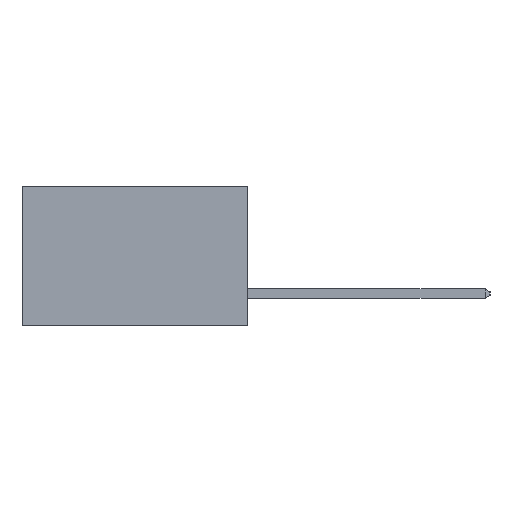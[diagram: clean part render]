
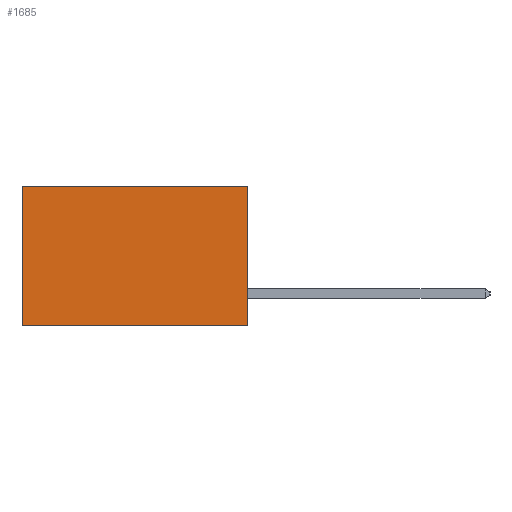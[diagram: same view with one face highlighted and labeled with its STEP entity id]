
A CAD part, left-side view. The second image highlights one B-rep face of the part: STEP entity #1685.
In plain terms, the highlighted planar face has unit normal (-1, 0, 0).
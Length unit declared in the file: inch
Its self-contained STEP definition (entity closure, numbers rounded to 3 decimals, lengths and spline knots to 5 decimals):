
#206 = VERTEX_POINT ( 'NONE', #11413 ) ;
#1685 = ADVANCED_FACE ( 'NONE', ( #15598 ), #6533, .F. ) ;
#3555 = VERTEX_POINT ( 'NONE', #18419 ) ;
#3852 = EDGE_CURVE ( 'NONE', #3555, #15900, #16230, .T. ) ;
#4130 = EDGE_CURVE ( 'NONE', #206, #18796, #12175, .T. ) ;
#6242 = DIRECTION ( 'NONE',  ( 1., 0., 0. ) ) ;
#6412 = DIRECTION ( 'NONE',  ( 0., 0., -1. ) ) ;
#6506 = CARTESIAN_POINT ( 'NONE',  ( 0.2615, 0., -0.37 ) ) ;
#6533 = PLANE ( 'NONE',  #6864 ) ;
#6864 = AXIS2_PLACEMENT_3D ( 'NONE', #6506, #6242, #6412 ) ;
#7263 = CARTESIAN_POINT ( 'NONE',  ( 0.2615, 0., -0.37 ) ) ;
#7342 = DIRECTION ( 'NONE',  ( 0., 0., -1. ) ) ;
#8049 = VECTOR ( 'NONE', #7342, 39.37008 ) ;
#8057 = VECTOR ( 'NONE', #14753, 39.37008 ) ;
#8686 = DIRECTION ( 'NONE',  ( 0., 1., 0. ) ) ;
#8915 = EDGE_CURVE ( 'NONE', #18796, #15900, #17696, .T. ) ;
#9102 = VECTOR ( 'NONE', #8686, 39.37008 ) ;
#9274 = ORIENTED_EDGE ( 'NONE', *, *, #16828, .T. ) ;
#9601 = LINE ( 'NONE', #13273, #9102 ) ;
#9613 = VECTOR ( 'NONE', #16079, 39.37008 ) ;
#10705 = ORIENTED_EDGE ( 'NONE', *, *, #8915, .F. ) ;
#11413 = CARTESIAN_POINT ( 'NONE',  ( 0.2615, 0., 0. ) ) ;
#12175 = LINE ( 'NONE', #7263, #8049 ) ;
#12704 = EDGE_LOOP ( 'NONE', ( #17351, #10705, #16142, #9274 ) ) ;
#13273 = CARTESIAN_POINT ( 'NONE',  ( 0.2615, 0., 0. ) ) ;
#14753 = DIRECTION ( 'NONE',  ( 0., 0., -1. ) ) ;
#14817 = CARTESIAN_POINT ( 'NONE',  ( 0.2615, 0.6, -0.37 ) ) ;
#15598 = FACE_OUTER_BOUND ( 'NONE', #12704, .T. ) ;
#15900 = VERTEX_POINT ( 'NONE', #17223 ) ;
#16079 = DIRECTION ( 'NONE',  ( 0., 1., 0. ) ) ;
#16142 = ORIENTED_EDGE ( 'NONE', *, *, #4130, .F. ) ;
#16179 = CARTESIAN_POINT ( 'NONE',  ( 0.2615, 0., -0.37 ) ) ;
#16230 = LINE ( 'NONE', #14817, #8057 ) ;
#16828 = EDGE_CURVE ( 'NONE', #206, #3555, #9601, .T. ) ;
#17223 = CARTESIAN_POINT ( 'NONE',  ( 0.2615, 0.6, -0.37 ) ) ;
#17351 = ORIENTED_EDGE ( 'NONE', *, *, #3852, .T. ) ;
#17367 = CARTESIAN_POINT ( 'NONE',  ( 0.2615, 0., -0.37 ) ) ;
#17696 = LINE ( 'NONE', #16179, #9613 ) ;
#18419 = CARTESIAN_POINT ( 'NONE',  ( 0.2615, 0.6, 0. ) ) ;
#18796 = VERTEX_POINT ( 'NONE', #17367 ) ;
